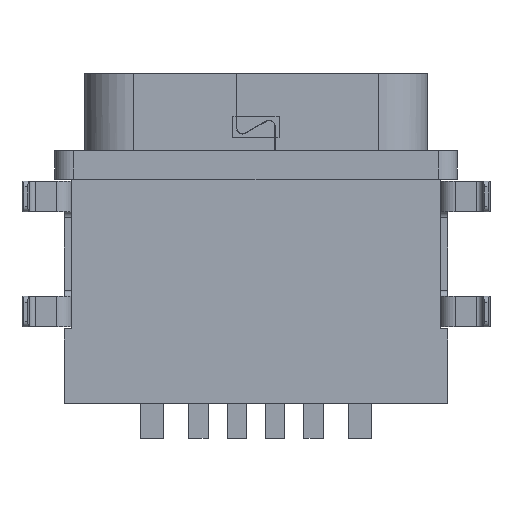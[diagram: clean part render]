
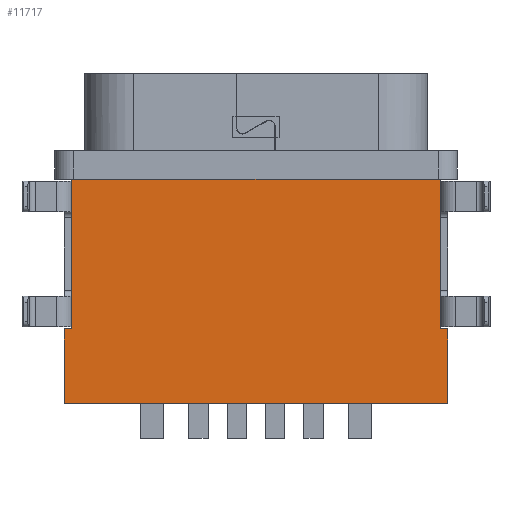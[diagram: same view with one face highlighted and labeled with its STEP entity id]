
A CAD part, front view. The second image highlights one B-rep face of the part: STEP entity #11717.
In plain terms, the highlighted face is planar.
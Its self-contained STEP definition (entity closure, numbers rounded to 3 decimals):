
#137 = LINE ( 'NONE', #7859, #960 ) ;
#371 = LINE ( 'NONE', #22944, #39507 ) ;
#960 = VECTOR ( 'NONE', #8479, 1000. ) ;
#1021 = LINE ( 'NONE', #22761, #40775 ) ;
#1392 = AXIS2_PLACEMENT_3D ( 'NONE', #20579, #20784, #29808 ) ;
#1943 = VERTEX_POINT ( 'NONE', #39345 ) ;
#2881 = CARTESIAN_POINT ( 'NONE',  ( 4.8, 5.75, -2.25 ) ) ;
#4160 = DIRECTION ( 'NONE',  ( 0., -1., 0. ) ) ;
#4217 = VECTOR ( 'NONE', #4160, 1000. ) ;
#4283 = FACE_OUTER_BOUND ( 'NONE', #13382, .T. ) ;
#4877 = LINE ( 'NONE', #14289, #21682 ) ;
#4980 = VERTEX_POINT ( 'NONE', #2881 ) ;
#7859 = CARTESIAN_POINT ( 'NONE',  ( 0., 7.7, -2.25 ) ) ;
#8038 = PLANE ( 'NONE',  #1392 ) ;
#8479 = DIRECTION ( 'NONE',  ( -1., 0., 0. ) ) ;
#8917 = CARTESIAN_POINT ( 'NONE',  ( 0., 5.75, -2.25 ) ) ;
#9389 = ORIENTED_EDGE ( 'NONE', *, *, #37207, .F. ) ;
#9638 = CARTESIAN_POINT ( 'NONE',  ( -4.8, 4.775, -2.25 ) ) ;
#10098 = ORIENTED_EDGE ( 'NONE', *, *, #30753, .F. ) ;
#10276 = LINE ( 'NONE', #9638, #32835 ) ;
#10447 = CARTESIAN_POINT ( 'NONE',  ( -5., 4.775, -2.25 ) ) ;
#11084 = ORIENTED_EDGE ( 'NONE', *, *, #40921, .F. ) ;
#11611 = ORIENTED_EDGE ( 'NONE', *, *, #40467, .F. ) ;
#11717 = ADVANCED_FACE ( 'NONE', ( #4283 ), #8038, .F. ) ;
#12690 = EDGE_CURVE ( 'NONE', #32763, #39898, #371, .T. ) ;
#12733 = VERTEX_POINT ( 'NONE', #34930 ) ;
#13099 = LINE ( 'NONE', #38609, #29663 ) ;
#13382 = EDGE_LOOP ( 'NONE', ( #22041, #29976, #16423, #11084, #37687, #9389, #10098, #11611 ) ) ;
#13902 = VERTEX_POINT ( 'NONE', #39972 ) ;
#14289 = CARTESIAN_POINT ( 'NONE',  ( 0., 1.85, -2.25 ) ) ;
#15015 = EDGE_CURVE ( 'NONE', #30308, #4980, #13099, .T. ) ;
#16423 = ORIENTED_EDGE ( 'NONE', *, *, #15015, .F. ) ;
#17926 = DIRECTION ( 'NONE',  ( 1., 0., 0. ) ) ;
#18388 = CARTESIAN_POINT ( 'NONE',  ( 5., 7.7, -2.25 ) ) ;
#18616 = VECTOR ( 'NONE', #17926, 1000. ) ;
#20579 = CARTESIAN_POINT ( 'NONE',  ( 5.2, 1.733, -2.25 ) ) ;
#20784 = DIRECTION ( 'NONE',  ( 0., 0., 1. ) ) ;
#21682 = VECTOR ( 'NONE', #30399, 1000. ) ;
#22041 = ORIENTED_EDGE ( 'NONE', *, *, #12690, .F. ) ;
#22307 = DIRECTION ( 'NONE',  ( 0., 1., 0. ) ) ;
#22761 = CARTESIAN_POINT ( 'NONE',  ( 0., 5.75, -2.25 ) ) ;
#22799 = DIRECTION ( 'NONE',  ( 0., -1., 0. ) ) ;
#22944 = CARTESIAN_POINT ( 'NONE',  ( 5., 4.775, -2.25 ) ) ;
#23188 = LINE ( 'NONE', #10447, #4217 ) ;
#24789 = VERTEX_POINT ( 'NONE', #30630 ) ;
#25485 = EDGE_CURVE ( 'NONE', #4980, #32763, #37578, .T. ) ;
#26038 = DIRECTION ( 'NONE',  ( 0., 1., 0. ) ) ;
#26516 = DIRECTION ( 'NONE',  ( 1., 0., 0. ) ) ;
#27934 = EDGE_CURVE ( 'NONE', #1943, #24789, #10276, .T. ) ;
#29663 = VECTOR ( 'NONE', #26038, 1000. ) ;
#29808 = DIRECTION ( 'NONE',  ( 0., 1., 0. ) ) ;
#29976 = ORIENTED_EDGE ( 'NONE', *, *, #25485, .F. ) ;
#30308 = VERTEX_POINT ( 'NONE', #31884 ) ;
#30399 = DIRECTION ( 'NONE',  ( 1., 0., 0. ) ) ;
#30630 = CARTESIAN_POINT ( 'NONE',  ( -4.8, 1.85, -2.25 ) ) ;
#30753 = EDGE_CURVE ( 'NONE', #12733, #13902, #23188, .T. ) ;
#31884 = CARTESIAN_POINT ( 'NONE',  ( 4.8, 1.85, -2.25 ) ) ;
#32763 = VERTEX_POINT ( 'NONE', #40780 ) ;
#32835 = VECTOR ( 'NONE', #22799, 1000. ) ;
#34930 = CARTESIAN_POINT ( 'NONE',  ( -5., 7.7, -2.25 ) ) ;
#37207 = EDGE_CURVE ( 'NONE', #13902, #1943, #1021, .T. ) ;
#37578 = LINE ( 'NONE', #8917, #18616 ) ;
#37687 = ORIENTED_EDGE ( 'NONE', *, *, #27934, .F. ) ;
#38609 = CARTESIAN_POINT ( 'NONE',  ( 4.8, 3.8, -2.25 ) ) ;
#39345 = CARTESIAN_POINT ( 'NONE',  ( -4.8, 5.75, -2.25 ) ) ;
#39507 = VECTOR ( 'NONE', #22307, 1000. ) ;
#39898 = VERTEX_POINT ( 'NONE', #18388 ) ;
#39972 = CARTESIAN_POINT ( 'NONE',  ( -5., 5.75, -2.25 ) ) ;
#40467 = EDGE_CURVE ( 'NONE', #39898, #12733, #137, .T. ) ;
#40775 = VECTOR ( 'NONE', #26516, 1000. ) ;
#40780 = CARTESIAN_POINT ( 'NONE',  ( 5., 5.75, -2.25 ) ) ;
#40921 = EDGE_CURVE ( 'NONE', #24789, #30308, #4877, .T. ) ;
